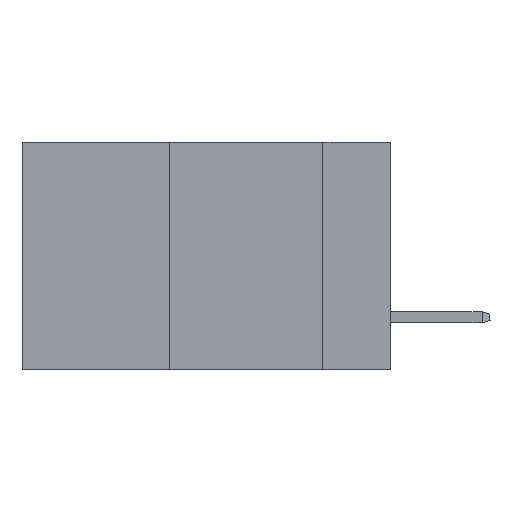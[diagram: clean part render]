
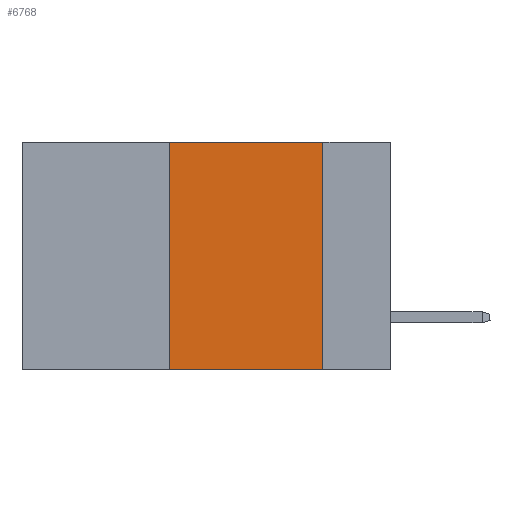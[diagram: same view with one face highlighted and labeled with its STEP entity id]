
A CAD part, left-side view. The second image highlights one B-rep face of the part: STEP entity #6768.
In plain terms, the highlighted planar face has unit normal (-1, 0, 0).
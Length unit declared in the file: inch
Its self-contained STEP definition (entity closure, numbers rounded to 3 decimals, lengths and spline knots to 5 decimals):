
#293 = DIRECTION ( 'NONE',  ( 1., 0., 0. ) ) ;
#1768 = EDGE_CURVE ( 'NONE', #38228, #45237, #36843, .T. ) ;
#3345 = LINE ( 'NONE', #40715, #48463 ) ;
#3980 = CARTESIAN_POINT ( 'NONE',  ( 0., 0.6, 0. ) ) ;
#6211 = AXIS2_PLACEMENT_3D ( 'NONE', #3980, #293, #31388 ) ;
#6768 = ADVANCED_FACE ( 'NONE', ( #25534 ), #33827, .F. ) ;
#7611 = CARTESIAN_POINT ( 'NONE',  ( 0., 0.36, 0. ) ) ;
#8593 = CARTESIAN_POINT ( 'NONE',  ( 0., 0.11, 0. ) ) ;
#8658 = LINE ( 'NONE', #23776, #14040 ) ;
#8992 = ORIENTED_EDGE ( 'NONE', *, *, #22680, .F. ) ;
#12445 = CARTESIAN_POINT ( 'NONE',  ( 0., 0.6, 0. ) ) ;
#12941 = VECTOR ( 'NONE', #35394, 39.37008 ) ;
#13000 = ORIENTED_EDGE ( 'NONE', *, *, #35014, .F. ) ;
#14006 = DIRECTION ( 'NONE',  ( 0., 0., 1. ) ) ;
#14040 = VECTOR ( 'NONE', #46855, 39.37008 ) ;
#22680 = EDGE_CURVE ( 'NONE', #45237, #32721, #35733, .T. ) ;
#23776 = CARTESIAN_POINT ( 'NONE',  ( 0., 0.6, -0.37 ) ) ;
#25534 = FACE_OUTER_BOUND ( 'NONE', #33789, .T. ) ;
#31388 = DIRECTION ( 'NONE',  ( 0., 0., -1. ) ) ;
#32003 = VECTOR ( 'NONE', #39284, 39.37008 ) ;
#32721 = VERTEX_POINT ( 'NONE', #36916 ) ;
#33789 = EDGE_LOOP ( 'NONE', ( #8992, #34100, #13000, #43558 ) ) ;
#33827 = PLANE ( 'NONE',  #6211 ) ;
#34100 = ORIENTED_EDGE ( 'NONE', *, *, #1768, .F. ) ;
#35014 = EDGE_CURVE ( 'NONE', #44856, #38228, #3345, .T. ) ;
#35394 = DIRECTION ( 'NONE',  ( 0., 0., -1. ) ) ;
#35733 = LINE ( 'NONE', #8593, #12941 ) ;
#36843 = LINE ( 'NONE', #12445, #32003 ) ;
#36916 = CARTESIAN_POINT ( 'NONE',  ( 0., 0.11, -0.37 ) ) ;
#38228 = VERTEX_POINT ( 'NONE', #7611 ) ;
#39284 = DIRECTION ( 'NONE',  ( 0., -1., 0. ) ) ;
#40715 = CARTESIAN_POINT ( 'NONE',  ( 0., 0.36, 0. ) ) ;
#40744 = EDGE_CURVE ( 'NONE', #44856, #32721, #8658, .T. ) ;
#43558 = ORIENTED_EDGE ( 'NONE', *, *, #40744, .T. ) ;
#44856 = VERTEX_POINT ( 'NONE', #47174 ) ;
#45237 = VERTEX_POINT ( 'NONE', #49186 ) ;
#46855 = DIRECTION ( 'NONE',  ( 0., -1., 0. ) ) ;
#47174 = CARTESIAN_POINT ( 'NONE',  ( 0., 0.36, -0.37 ) ) ;
#48463 = VECTOR ( 'NONE', #14006, 39.37008 ) ;
#49186 = CARTESIAN_POINT ( 'NONE',  ( 0., 0.11, 0. ) ) ;
